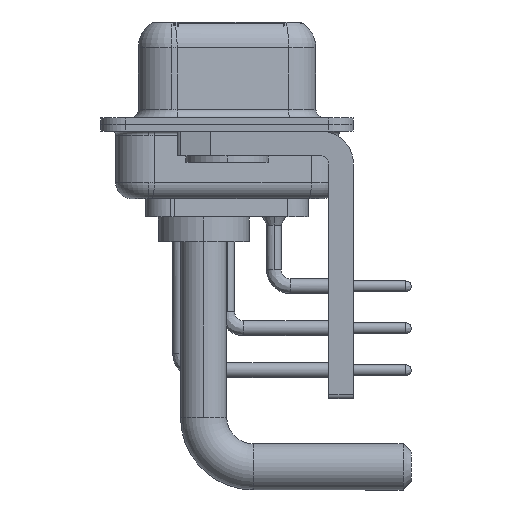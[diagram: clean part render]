
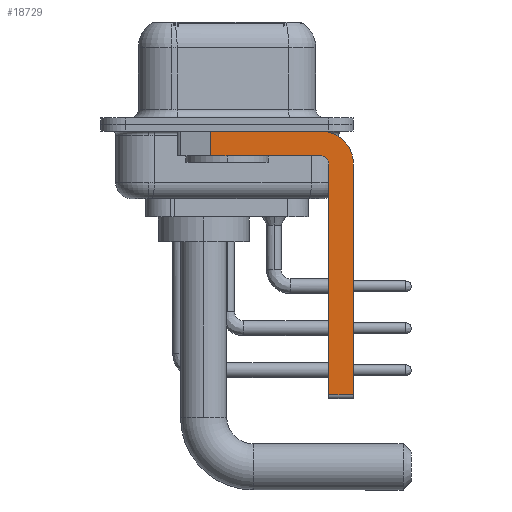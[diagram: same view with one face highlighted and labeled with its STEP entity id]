
A CAD part, left-side view. The second image highlights one B-rep face of the part: STEP entity #18729.
In plain terms, the highlighted planar face has unit normal (-1, 0, 0).
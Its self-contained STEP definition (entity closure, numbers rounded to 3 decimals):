
#83 = VERTEX_POINT ( 'NONE', #4728 ) ;
#520 = EDGE_LOOP ( 'NONE', ( #13256, #8121, #8531, #30282, #13098, #25951, #14580, #18935 ) ) ;
#955 = EDGE_CURVE ( 'NONE', #8964, #21484, #4118, .T. ) ;
#1504 = EDGE_CURVE ( 'NONE', #11490, #5475, #10695, .T. ) ;
#3006 = DIRECTION ( 'NONE',  ( 0., 0., -1. ) ) ;
#4118 = LINE ( 'NONE', #9742, #17214 ) ;
#4326 = CARTESIAN_POINT ( 'NONE',  ( -2.9, -5.65, -16.35 ) ) ;
#4728 = CARTESIAN_POINT ( 'NONE',  ( -2.9, 0.978, -1.9 ) ) ;
#4920 = AXIS2_PLACEMENT_3D ( 'NONE', #9879, #31458, #31290 ) ;
#5109 = CARTESIAN_POINT ( 'NONE',  ( -2.9, -5.65, -2.4 ) ) ;
#5475 = VERTEX_POINT ( 'NONE', #7044 ) ;
#7044 = CARTESIAN_POINT ( 'NONE',  ( -2.9, -5.65, -0.4 ) ) ;
#7892 = DIRECTION ( 'NONE',  ( 0., -1., 0. ) ) ;
#8121 = ORIENTED_EDGE ( 'NONE', *, *, #22057, .T. ) ;
#8273 = CARTESIAN_POINT ( 'NONE',  ( -2.9, -5.65, -1.9 ) ) ;
#8531 = ORIENTED_EDGE ( 'NONE', *, *, #34354, .F. ) ;
#8964 = VERTEX_POINT ( 'NONE', #18637 ) ;
#9436 = DIRECTION ( 'NONE',  ( 0., -1., 0. ) ) ;
#9742 = CARTESIAN_POINT ( 'NONE',  ( -2.9, -6.15, -16.6 ) ) ;
#9791 = VERTEX_POINT ( 'NONE', #33916 ) ;
#9801 = EDGE_CURVE ( 'NONE', #21484, #30571, #18395, .T. ) ;
#9879 = CARTESIAN_POINT ( 'NONE',  ( -2.9, -5.65, -2.4 ) ) ;
#10534 = DIRECTION ( 'NONE',  ( 0., 0., -1. ) ) ;
#10695 = LINE ( 'NONE', #21065, #26870 ) ;
#11090 = FACE_OUTER_BOUND ( 'NONE', #520, .T. ) ;
#11490 = VERTEX_POINT ( 'NONE', #29581 ) ;
#11945 = EDGE_CURVE ( 'NONE', #5475, #12480, #33083, .T. ) ;
#12480 = VERTEX_POINT ( 'NONE', #32152 ) ;
#13098 = ORIENTED_EDGE ( 'NONE', *, *, #955, .F. ) ;
#13256 = ORIENTED_EDGE ( 'NONE', *, *, #1504, .F. ) ;
#14116 = CARTESIAN_POINT ( 'NONE',  ( -2.9, -5.65, -2.4 ) ) ;
#14580 = ORIENTED_EDGE ( 'NONE', *, *, #21071, .F. ) ;
#14913 = AXIS2_PLACEMENT_3D ( 'NONE', #5109, #23914, #3006 ) ;
#15489 = VECTOR ( 'NONE', #18975, 1000. ) ;
#16185 = VECTOR ( 'NONE', #10534, 1000. ) ;
#17214 = VECTOR ( 'NONE', #25563, 1000. ) ;
#17870 = VECTOR ( 'NONE', #25978, 1000. ) ;
#18395 = CIRCLE ( 'NONE', #4920, 0.5 ) ;
#18454 = CARTESIAN_POINT ( 'NONE',  ( -2.9, 0.978, -1.9 ) ) ;
#18568 = VECTOR ( 'NONE', #9436, 1000. ) ;
#18637 = CARTESIAN_POINT ( 'NONE',  ( -2.9, -6.15, -16.35 ) ) ;
#18729 = ADVANCED_FACE ( 'NONE', ( #11090 ), #29711, .F. ) ;
#18935 = ORIENTED_EDGE ( 'NONE', *, *, #11945, .F. ) ;
#18975 = DIRECTION ( 'NONE',  ( 0., 1., 0. ) ) ;
#19149 = LINE ( 'NONE', #8273, #15489 ) ;
#21065 = CARTESIAN_POINT ( 'NONE',  ( -2.9, 3., -0.4 ) ) ;
#21071 = EDGE_CURVE ( 'NONE', #12480, #9791, #30694, .T. ) ;
#21484 = VERTEX_POINT ( 'NONE', #31643 ) ;
#22057 = EDGE_CURVE ( 'NONE', #11490, #83, #26530, .T. ) ;
#23914 = DIRECTION ( 'NONE',  ( 1., 0., 0. ) ) ;
#24309 = EDGE_CURVE ( 'NONE', #8964, #9791, #25605, .T. ) ;
#24828 = DIRECTION ( 'NONE',  ( 1., 0., 0. ) ) ;
#25249 = AXIS2_PLACEMENT_3D ( 'NONE', #14116, #24828, #32545 ) ;
#25563 = DIRECTION ( 'NONE',  ( 0., 0., 1. ) ) ;
#25605 = LINE ( 'NONE', #4326, #18568 ) ;
#25951 = ORIENTED_EDGE ( 'NONE', *, *, #24309, .T. ) ;
#25978 = DIRECTION ( 'NONE',  ( 0., 0., -1. ) ) ;
#26530 = LINE ( 'NONE', #18454, #16185 ) ;
#26870 = VECTOR ( 'NONE', #7892, 1000. ) ;
#29581 = CARTESIAN_POINT ( 'NONE',  ( -2.9, 0.978, -0.4 ) ) ;
#29711 = PLANE ( 'NONE',  #14913 ) ;
#30282 = ORIENTED_EDGE ( 'NONE', *, *, #9801, .F. ) ;
#30571 = VERTEX_POINT ( 'NONE', #31561 ) ;
#30694 = LINE ( 'NONE', #30873, #17870 ) ;
#30873 = CARTESIAN_POINT ( 'NONE',  ( -2.9, -7.65, -2.4 ) ) ;
#31290 = DIRECTION ( 'NONE',  ( 0., 0., 1. ) ) ;
#31458 = DIRECTION ( 'NONE',  ( -1., 0., 0. ) ) ;
#31561 = CARTESIAN_POINT ( 'NONE',  ( -2.9, -5.65, -1.9 ) ) ;
#31643 = CARTESIAN_POINT ( 'NONE',  ( -2.9, -6.15, -2.4 ) ) ;
#32152 = CARTESIAN_POINT ( 'NONE',  ( -2.9, -7.65, -2.4 ) ) ;
#32545 = DIRECTION ( 'NONE',  ( 0., 0., -1. ) ) ;
#33083 = CIRCLE ( 'NONE', #25249, 2. ) ;
#33916 = CARTESIAN_POINT ( 'NONE',  ( -2.9, -7.65, -16.35 ) ) ;
#34354 = EDGE_CURVE ( 'NONE', #30571, #83, #19149, .T. ) ;
